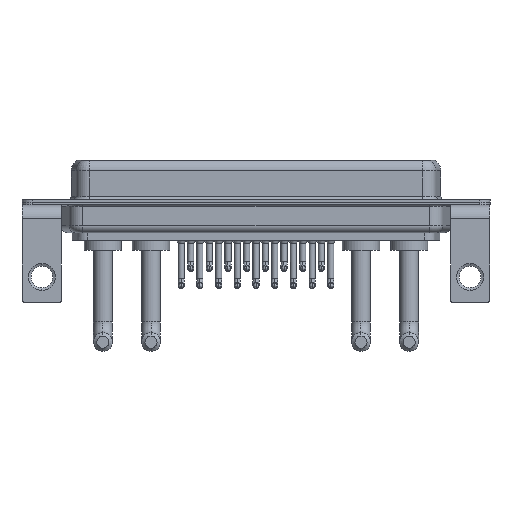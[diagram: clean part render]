
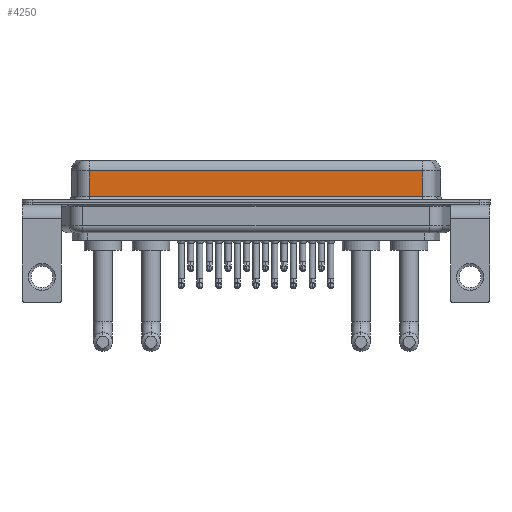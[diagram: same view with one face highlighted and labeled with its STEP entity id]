
A CAD part, front view. The second image highlights one B-rep face of the part: STEP entity #4250.
In plain terms, the highlighted planar face has unit normal (0, -1, 0).
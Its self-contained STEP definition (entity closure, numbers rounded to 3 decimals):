
#1017 = LINE ( 'NONE', #11612, #9957 ) ;
#1212 = VERTEX_POINT ( 'NONE', #16736 ) ;
#1229 = DIRECTION ( 'NONE',  ( 0., 0., 1. ) ) ;
#1514 = VERTEX_POINT ( 'NONE', #16356 ) ;
#1761 = LINE ( 'NONE', #1877, #5465 ) ;
#1877 = CARTESIAN_POINT ( 'NONE',  ( 7.038, -3.95, 6.4 ) ) ;
#3347 = VERTEX_POINT ( 'NONE', #22730 ) ;
#3969 = ORIENTED_EDGE ( 'NONE', *, *, #16286, .T. ) ;
#4250 = ADVANCED_FACE ( 'NONE', ( #19055 ), #6860, .F. ) ;
#5465 = VECTOR ( 'NONE', #13737, 1000. ) ;
#5822 = CARTESIAN_POINT ( 'NONE',  ( 56.462, -3.95, 6.4 ) ) ;
#6317 = ORIENTED_EDGE ( 'NONE', *, *, #7135, .T. ) ;
#6860 = PLANE ( 'NONE',  #14142 ) ;
#7135 = EDGE_CURVE ( 'NONE', #1514, #21173, #15970, .T. ) ;
#8371 = DIRECTION ( 'NONE',  ( 0., 1., 0. ) ) ;
#9716 = EDGE_LOOP ( 'NONE', ( #14321, #6317, #13203, #3969 ) ) ;
#9957 = VECTOR ( 'NONE', #14961, 1000. ) ;
#10533 = CARTESIAN_POINT ( 'NONE',  ( 56.462, -3.95, 6.4 ) ) ;
#11612 = CARTESIAN_POINT ( 'NONE',  ( 56.462, -3.95, 0.9 ) ) ;
#12963 = LINE ( 'NONE', #5822, #22407 ) ;
#12975 = CARTESIAN_POINT ( 'NONE',  ( 56.462, -3.95, 4.65 ) ) ;
#13075 = DIRECTION ( 'NONE',  ( 0., 0., -1. ) ) ;
#13203 = ORIENTED_EDGE ( 'NONE', *, *, #14654, .T. ) ;
#13737 = DIRECTION ( 'NONE',  ( 0., 0., -1. ) ) ;
#14142 = AXIS2_PLACEMENT_3D ( 'NONE', #10533, #8371, #1229 ) ;
#14321 = ORIENTED_EDGE ( 'NONE', *, *, #20193, .F. ) ;
#14654 = EDGE_CURVE ( 'NONE', #21173, #3347, #1761, .T. ) ;
#14833 = CARTESIAN_POINT ( 'NONE',  ( 7.038, -3.95, 4.65 ) ) ;
#14961 = DIRECTION ( 'NONE',  ( 1., 0., 0. ) ) ;
#15970 = LINE ( 'NONE', #12975, #20720 ) ;
#16286 = EDGE_CURVE ( 'NONE', #3347, #1212, #1017, .T. ) ;
#16356 = CARTESIAN_POINT ( 'NONE',  ( 56.462, -3.95, 4.65 ) ) ;
#16736 = CARTESIAN_POINT ( 'NONE',  ( 56.462, -3.95, 0.9 ) ) ;
#19055 = FACE_OUTER_BOUND ( 'NONE', #9716, .T. ) ;
#19972 = DIRECTION ( 'NONE',  ( -1., 0., 0. ) ) ;
#20193 = EDGE_CURVE ( 'NONE', #1514, #1212, #12963, .T. ) ;
#20720 = VECTOR ( 'NONE', #19972, 1000. ) ;
#21173 = VERTEX_POINT ( 'NONE', #14833 ) ;
#22407 = VECTOR ( 'NONE', #13075, 1000. ) ;
#22730 = CARTESIAN_POINT ( 'NONE',  ( 7.038, -3.95, 0.9 ) ) ;
